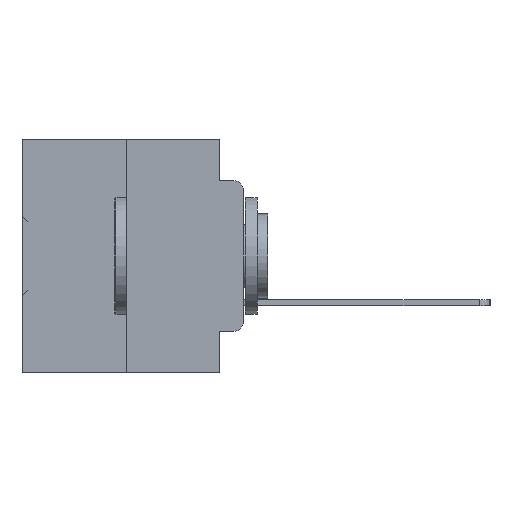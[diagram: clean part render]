
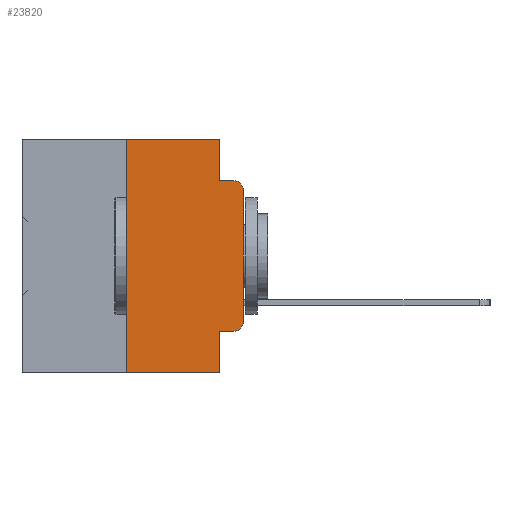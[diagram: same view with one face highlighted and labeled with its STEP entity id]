
A CAD part, left-side view. The second image highlights one B-rep face of the part: STEP entity #23820.
In plain terms, the highlighted planar face has unit normal (-1, 0, 0).
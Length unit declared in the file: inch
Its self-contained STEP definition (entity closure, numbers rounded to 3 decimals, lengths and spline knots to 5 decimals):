
#317 = EDGE_CURVE ( 'NONE', #18871, #5997, #21074, .T. ) ;
#474 = VECTOR ( 'NONE', #28568, 39.37008 ) ;
#1660 = VECTOR ( 'NONE', #13143, 39.37008 ) ;
#2567 = ORIENTED_EDGE ( 'NONE', *, *, #6256, .T. ) ;
#2831 = VERTEX_POINT ( 'NONE', #31182 ) ;
#2929 = EDGE_LOOP ( 'NONE', ( #2567, #17524, #3333, #6106, #8945, #36207, #7080, #32629, #36709, #31750 ) ) ;
#2932 = CARTESIAN_POINT ( 'NONE',  ( 0., 0.051, -0.4115 ) ) ;
#3333 = ORIENTED_EDGE ( 'NONE', *, *, #317, .F. ) ;
#4254 = EDGE_CURVE ( 'NONE', #25233, #5997, #7531, .T. ) ;
#5102 = LINE ( 'NONE', #22510, #6047 ) ;
#5997 = VERTEX_POINT ( 'NONE', #17688 ) ;
#6047 = VECTOR ( 'NONE', #37156, 39.37008 ) ;
#6106 = ORIENTED_EDGE ( 'NONE', *, *, #32867, .F. ) ;
#6256 = EDGE_CURVE ( 'NONE', #2831, #25233, #8362, .T. ) ;
#7080 = ORIENTED_EDGE ( 'NONE', *, *, #37221, .T. ) ;
#7239 = CARTESIAN_POINT ( 'NONE',  ( 0., 0.25, 0. ) ) ;
#7322 = CARTESIAN_POINT ( 'NONE',  ( 0., 0.473, -0.5 ) ) ;
#7531 = CIRCLE ( 'NONE', #28340, 0.02 ) ;
#8362 = LINE ( 'NONE', #10729, #474 ) ;
#8945 = ORIENTED_EDGE ( 'NONE', *, *, #21331, .F. ) ;
#9664 = LINE ( 'NONE', #2932, #25542 ) ;
#9709 = CARTESIAN_POINT ( 'NONE',  ( 0., 0.02, -0.1085 ) ) ;
#9999 = VERTEX_POINT ( 'NONE', #26852 ) ;
#10291 = CARTESIAN_POINT ( 'NONE',  ( 0., 0.051, 0. ) ) ;
#10729 = CARTESIAN_POINT ( 'NONE',  ( 0., 0., 0. ) ) ;
#11761 = DIRECTION ( 'NONE',  ( 0., -1., 0. ) ) ;
#12292 = DIRECTION ( 'NONE',  ( -1., 0., 0. ) ) ;
#12373 = PLANE ( 'NONE',  #13574 ) ;
#12677 = DIRECTION ( 'NONE',  ( 0., 0., -1. ) ) ;
#12845 = LINE ( 'NONE', #7322, #19874 ) ;
#13026 = VERTEX_POINT ( 'NONE', #18583 ) ;
#13120 = LINE ( 'NONE', #34201, #28053 ) ;
#13143 = DIRECTION ( 'NONE',  ( 0., 0., -1. ) ) ;
#13262 = CARTESIAN_POINT ( 'NONE',  ( 0., 0.051, -0.0885 ) ) ;
#13574 = AXIS2_PLACEMENT_3D ( 'NONE', #24417, #33232, #15465 ) ;
#14941 = VERTEX_POINT ( 'NONE', #7239 ) ;
#15465 = DIRECTION ( 'NONE',  ( 0., 0., -1. ) ) ;
#15663 = CARTESIAN_POINT ( 'NONE',  ( 0., 0.051, -0.5 ) ) ;
#16508 = CARTESIAN_POINT ( 'NONE',  ( 0., 0.25, 0. ) ) ;
#17500 = LINE ( 'NONE', #10291, #1660 ) ;
#17524 = ORIENTED_EDGE ( 'NONE', *, *, #4254, .T. ) ;
#17688 = CARTESIAN_POINT ( 'NONE',  ( 0., 0.02, -0.0885 ) ) ;
#18583 = CARTESIAN_POINT ( 'NONE',  ( 0., 0.051, -0.4115 ) ) ;
#18871 = VERTEX_POINT ( 'NONE', #28342 ) ;
#19187 = DIRECTION ( 'NONE',  ( 0., -1., 0. ) ) ;
#19874 = VECTOR ( 'NONE', #19187, 39.37008 ) ;
#20198 = CARTESIAN_POINT ( 'NONE',  ( 0., 0., -0.1085 ) ) ;
#21044 = EDGE_CURVE ( 'NONE', #29800, #2831, #24322, .T. ) ;
#21074 = LINE ( 'NONE', #13262, #35723 ) ;
#21331 = EDGE_CURVE ( 'NONE', #14941, #36243, #5102, .T. ) ;
#22510 = CARTESIAN_POINT ( 'NONE',  ( 0., 0.473, 0. ) ) ;
#23054 = EDGE_CURVE ( 'NONE', #13026, #29800, #9664, .T. ) ;
#23820 = ADVANCED_FACE ( 'NONE', ( #28233 ), #12373, .F. ) ;
#24322 = CIRCLE ( 'NONE', #38223, 0.02 ) ;
#24417 = CARTESIAN_POINT ( 'NONE',  ( 0., 0.473, 0. ) ) ;
#25033 = EDGE_CURVE ( 'NONE', #13026, #35219, #17500, .T. ) ;
#25233 = VERTEX_POINT ( 'NONE', #20198 ) ;
#25542 = VECTOR ( 'NONE', #35426, 39.37008 ) ;
#26852 = CARTESIAN_POINT ( 'NONE',  ( 0., 0.25, -0.5 ) ) ;
#28053 = VECTOR ( 'NONE', #37077, 39.37008 ) ;
#28233 = FACE_OUTER_BOUND ( 'NONE', #2929, .T. ) ;
#28340 = AXIS2_PLACEMENT_3D ( 'NONE', #9709, #30500, #12677 ) ;
#28342 = CARTESIAN_POINT ( 'NONE',  ( 0., 0.051, -0.0885 ) ) ;
#28568 = DIRECTION ( 'NONE',  ( 0., 0., 1. ) ) ;
#28951 = EDGE_CURVE ( 'NONE', #9999, #14941, #31132, .T. ) ;
#29800 = VERTEX_POINT ( 'NONE', #35774 ) ;
#30101 = CARTESIAN_POINT ( 'NONE',  ( 0., 0.02, -0.3915 ) ) ;
#30500 = DIRECTION ( 'NONE',  ( -1., 0., 0. ) ) ;
#31132 = LINE ( 'NONE', #16508, #36980 ) ;
#31182 = CARTESIAN_POINT ( 'NONE',  ( 0., 0., -0.3915 ) ) ;
#31312 = DIRECTION ( 'NONE',  ( 0., 0., 1. ) ) ;
#31750 = ORIENTED_EDGE ( 'NONE', *, *, #21044, .T. ) ;
#32629 = ORIENTED_EDGE ( 'NONE', *, *, #25033, .F. ) ;
#32867 = EDGE_CURVE ( 'NONE', #36243, #18871, #13120, .T. ) ;
#33029 = DIRECTION ( 'NONE',  ( 0., 0., -1. ) ) ;
#33232 = DIRECTION ( 'NONE',  ( 1., 0., 0. ) ) ;
#34201 = CARTESIAN_POINT ( 'NONE',  ( 0., 0.051, 0. ) ) ;
#35219 = VERTEX_POINT ( 'NONE', #15663 ) ;
#35354 = CARTESIAN_POINT ( 'NONE',  ( 0., 0.051, 0. ) ) ;
#35426 = DIRECTION ( 'NONE',  ( 0., -1., 0. ) ) ;
#35723 = VECTOR ( 'NONE', #11761, 39.37008 ) ;
#35774 = CARTESIAN_POINT ( 'NONE',  ( 0., 0.02, -0.4115 ) ) ;
#36207 = ORIENTED_EDGE ( 'NONE', *, *, #28951, .F. ) ;
#36243 = VERTEX_POINT ( 'NONE', #35354 ) ;
#36709 = ORIENTED_EDGE ( 'NONE', *, *, #23054, .T. ) ;
#36980 = VECTOR ( 'NONE', #31312, 39.37008 ) ;
#37077 = DIRECTION ( 'NONE',  ( 0., 0., -1. ) ) ;
#37156 = DIRECTION ( 'NONE',  ( 0., -1., 0. ) ) ;
#37221 = EDGE_CURVE ( 'NONE', #9999, #35219, #12845, .T. ) ;
#38223 = AXIS2_PLACEMENT_3D ( 'NONE', #30101, #12292, #33029 ) ;
